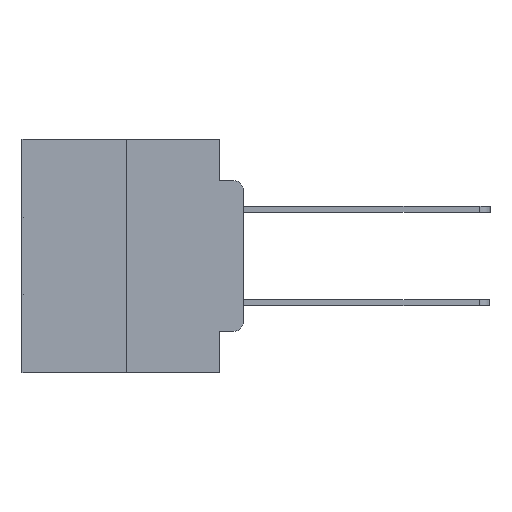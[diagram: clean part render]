
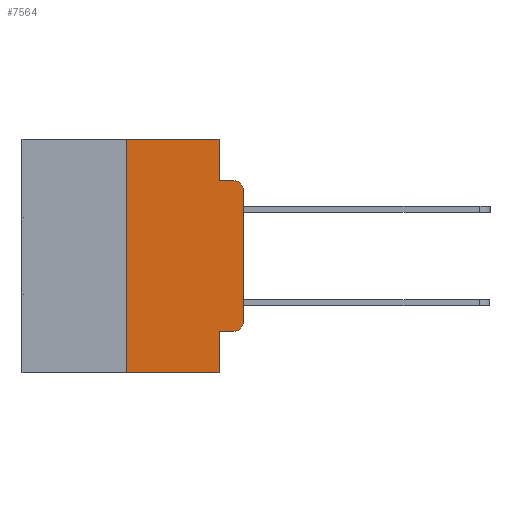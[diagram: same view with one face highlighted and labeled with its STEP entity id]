
A CAD part, left-side view. The second image highlights one B-rep face of the part: STEP entity #7564.
In plain terms, the highlighted planar face has unit normal (-1, 0, 0).
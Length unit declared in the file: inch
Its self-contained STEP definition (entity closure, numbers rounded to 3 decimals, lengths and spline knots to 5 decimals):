
#1 = VECTOR ( 'NONE', #3525, 39.37008 ) ;
#696 = CIRCLE ( 'NONE', #6872, 0.02 ) ;
#1403 = CARTESIAN_POINT ( 'NONE',  ( 0., 0.25, 0. ) ) ;
#1751 = LINE ( 'NONE', #9922, #18039 ) ;
#1769 = ORIENTED_EDGE ( 'NONE', *, *, #29276, .F. ) ;
#1824 = VERTEX_POINT ( 'NONE', #3005 ) ;
#2087 = DIRECTION ( 'NONE',  ( -1., 0., 0. ) ) ;
#2654 = CIRCLE ( 'NONE', #11135, 0.02 ) ;
#2671 = VERTEX_POINT ( 'NONE', #21700 ) ;
#3005 = CARTESIAN_POINT ( 'NONE',  ( 0., 0.051, -0.5 ) ) ;
#3525 = DIRECTION ( 'NONE',  ( 0., 0., -1. ) ) ;
#3577 = VERTEX_POINT ( 'NONE', #26345 ) ;
#3669 = CARTESIAN_POINT ( 'NONE',  ( 0., 0.02, -0.4115 ) ) ;
#3817 = EDGE_CURVE ( 'NONE', #16812, #14010, #1751, .T. ) ;
#4967 = DIRECTION ( 'NONE',  ( 0., 0., -1. ) ) ;
#5141 = CARTESIAN_POINT ( 'NONE',  ( 0., 0.25, 0. ) ) ;
#5143 = VECTOR ( 'NONE', #4967, 39.37008 ) ;
#5411 = VECTOR ( 'NONE', #26547, 39.37008 ) ;
#5564 = LINE ( 'NONE', #28650, #11739 ) ;
#5644 = LINE ( 'NONE', #25442, #15927 ) ;
#6872 = AXIS2_PLACEMENT_3D ( 'NONE', #15988, #2087, #18256 ) ;
#7564 = ADVANCED_FACE ( 'NONE', ( #15263 ), #27730, .F. ) ;
#8150 = ORIENTED_EDGE ( 'NONE', *, *, #23338, .F. ) ;
#8368 = CARTESIAN_POINT ( 'NONE',  ( 0., 0.051, -0.0885 ) ) ;
#8799 = CARTESIAN_POINT ( 'NONE',  ( 0., 0.473, 0. ) ) ;
#9581 = ORIENTED_EDGE ( 'NONE', *, *, #21840, .F. ) ;
#9582 = CARTESIAN_POINT ( 'NONE',  ( 0., 0.051, 0. ) ) ;
#9922 = CARTESIAN_POINT ( 'NONE',  ( 0., 0., 0. ) ) ;
#10871 = CARTESIAN_POINT ( 'NONE',  ( 0., 0.02, -0.0885 ) ) ;
#10898 = DIRECTION ( 'NONE',  ( -1., 0., 0. ) ) ;
#11022 = ORIENTED_EDGE ( 'NONE', *, *, #20334, .F. ) ;
#11135 = AXIS2_PLACEMENT_3D ( 'NONE', #24417, #10898, #26623 ) ;
#11322 = LINE ( 'NONE', #9582, #5143 ) ;
#11739 = VECTOR ( 'NONE', #24192, 39.37008 ) ;
#11802 = LINE ( 'NONE', #8799, #28990 ) ;
#11955 = DIRECTION ( 'NONE',  ( 0., -1., 0. ) ) ;
#12182 = EDGE_CURVE ( 'NONE', #14010, #12755, #2654, .T. ) ;
#12272 = CARTESIAN_POINT ( 'NONE',  ( 0., 0.051, -0.0885 ) ) ;
#12755 = VERTEX_POINT ( 'NONE', #10871 ) ;
#12910 = EDGE_CURVE ( 'NONE', #21222, #16812, #696, .T. ) ;
#13083 = VERTEX_POINT ( 'NONE', #5141 ) ;
#13133 = ORIENTED_EDGE ( 'NONE', *, *, #12910, .T. ) ;
#14010 = VERTEX_POINT ( 'NONE', #23533 ) ;
#14347 = EDGE_CURVE ( 'NONE', #13083, #2671, #11802, .T. ) ;
#14539 = DIRECTION ( 'NONE',  ( 0., -1., 0. ) ) ;
#14549 = EDGE_LOOP ( 'NONE', ( #28569, #24065, #1769, #8150, #20217, #9581, #15606, #11022, #17014, #13133 ) ) ;
#15192 = DIRECTION ( 'NONE',  ( 0., 0., -1. ) ) ;
#15263 = FACE_OUTER_BOUND ( 'NONE', #14549, .T. ) ;
#15606 = ORIENTED_EDGE ( 'NONE', *, *, #23777, .T. ) ;
#15927 = VECTOR ( 'NONE', #11955, 39.37008 ) ;
#15988 = CARTESIAN_POINT ( 'NONE',  ( 0., 0.02, -0.3915 ) ) ;
#16115 = CARTESIAN_POINT ( 'NONE',  ( 0., 0.051, -0.4115 ) ) ;
#16812 = VERTEX_POINT ( 'NONE', #18627 ) ;
#17014 = ORIENTED_EDGE ( 'NONE', *, *, #29443, .T. ) ;
#17305 = CARTESIAN_POINT ( 'NONE',  ( 0., 0.051, 0. ) ) ;
#17413 = VERTEX_POINT ( 'NONE', #16115 ) ;
#18039 = VECTOR ( 'NONE', #29056, 39.37008 ) ;
#18256 = DIRECTION ( 'NONE',  ( 0., 0., -1. ) ) ;
#18627 = CARTESIAN_POINT ( 'NONE',  ( 0., 0., -0.3915 ) ) ;
#20217 = ORIENTED_EDGE ( 'NONE', *, *, #14347, .F. ) ;
#20334 = EDGE_CURVE ( 'NONE', #17413, #1824, #11322, .T. ) ;
#20619 = VERTEX_POINT ( 'NONE', #8368 ) ;
#21222 = VERTEX_POINT ( 'NONE', #3669 ) ;
#21409 = CARTESIAN_POINT ( 'NONE',  ( 0., 0.473, 0. ) ) ;
#21700 = CARTESIAN_POINT ( 'NONE',  ( 0., 0.051, 0. ) ) ;
#21840 = EDGE_CURVE ( 'NONE', #3577, #13083, #23587, .T. ) ;
#22008 = VECTOR ( 'NONE', #14539, 39.37008 ) ;
#22356 = DIRECTION ( 'NONE',  ( 0., -1., 0. ) ) ;
#23338 = EDGE_CURVE ( 'NONE', #2671, #20619, #29026, .T. ) ;
#23533 = CARTESIAN_POINT ( 'NONE',  ( 0., 0., -0.1085 ) ) ;
#23587 = LINE ( 'NONE', #1403, #5411 ) ;
#23777 = EDGE_CURVE ( 'NONE', #3577, #1824, #5644, .T. ) ;
#24065 = ORIENTED_EDGE ( 'NONE', *, *, #12182, .T. ) ;
#24192 = DIRECTION ( 'NONE',  ( 0., -1., 0. ) ) ;
#24417 = CARTESIAN_POINT ( 'NONE',  ( 0., 0.02, -0.1085 ) ) ;
#25442 = CARTESIAN_POINT ( 'NONE',  ( 0., 0.473, -0.5 ) ) ;
#26345 = CARTESIAN_POINT ( 'NONE',  ( 0., 0.25, -0.5 ) ) ;
#26547 = DIRECTION ( 'NONE',  ( 0., 0., 1. ) ) ;
#26623 = DIRECTION ( 'NONE',  ( 0., 0., -1. ) ) ;
#27730 = PLANE ( 'NONE',  #29638 ) ;
#28569 = ORIENTED_EDGE ( 'NONE', *, *, #3817, .T. ) ;
#28614 = LINE ( 'NONE', #12272, #22008 ) ;
#28650 = CARTESIAN_POINT ( 'NONE',  ( 0., 0.051, -0.4115 ) ) ;
#28911 = DIRECTION ( 'NONE',  ( 1., 0., 0. ) ) ;
#28990 = VECTOR ( 'NONE', #22356, 39.37008 ) ;
#29026 = LINE ( 'NONE', #17305, #1 ) ;
#29056 = DIRECTION ( 'NONE',  ( 0., 0., 1. ) ) ;
#29276 = EDGE_CURVE ( 'NONE', #20619, #12755, #28614, .T. ) ;
#29443 = EDGE_CURVE ( 'NONE', #17413, #21222, #5564, .T. ) ;
#29638 = AXIS2_PLACEMENT_3D ( 'NONE', #21409, #28911, #15192 ) ;
